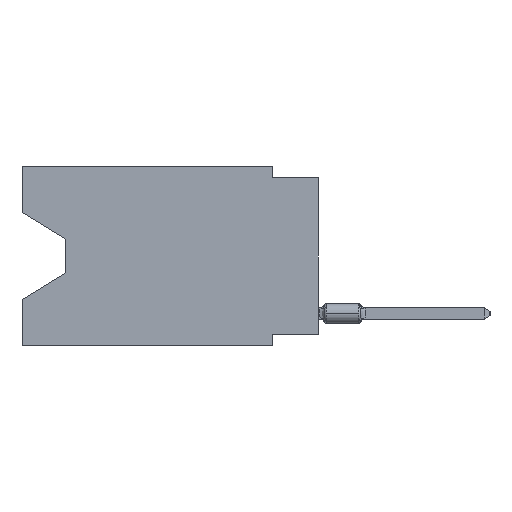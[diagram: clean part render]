
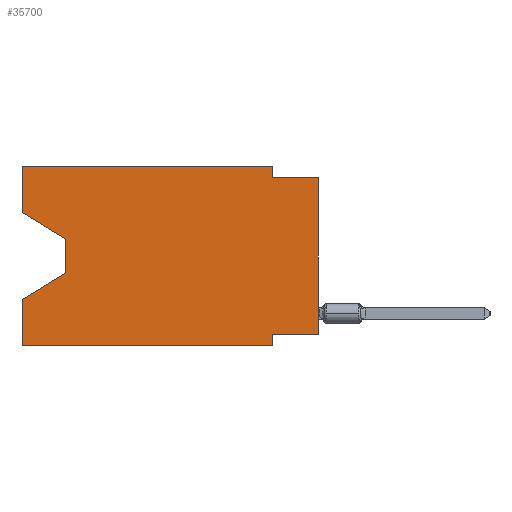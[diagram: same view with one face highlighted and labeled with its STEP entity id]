
A CAD part, left-side view. The second image highlights one B-rep face of the part: STEP entity #35700.
In plain terms, the highlighted planar face has unit normal (-1, 0, 0).
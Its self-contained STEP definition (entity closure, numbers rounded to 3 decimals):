
#218 = VERTEX_POINT ( 'NONE', #28616 ) ;
#376 = ORIENTED_EDGE ( 'NONE', *, *, #25564, .F. ) ;
#416 = CARTESIAN_POINT ( 'NONE',  ( 0., 2.54, -9.906 ) ) ;
#848 = LINE ( 'NONE', #58974, #63170 ) ;
#940 = DIRECTION ( 'NONE',  ( 0., -0.855, -0.519 ) ) ;
#2108 = VERTEX_POINT ( 'NONE', #58281 ) ;
#2671 = VERTEX_POINT ( 'NONE', #14211 ) ;
#4858 = CARTESIAN_POINT ( 'NONE',  ( 0., 13.97, -4.013 ) ) ;
#4919 = VECTOR ( 'NONE', #16366, 1000. ) ;
#5363 = DIRECTION ( 'NONE',  ( 0., 0., -1. ) ) ;
#5386 = LINE ( 'NONE', #6330, #28472 ) ;
#5789 = LINE ( 'NONE', #11554, #56213 ) ;
#6099 = CARTESIAN_POINT ( 'NONE',  ( 0., 0., 0. ) ) ;
#6330 = CARTESIAN_POINT ( 'NONE',  ( 0., 13.97, -5.893 ) ) ;
#7498 = VERTEX_POINT ( 'NONE', #21875 ) ;
#8392 = CARTESIAN_POINT ( 'NONE',  ( 0., 16.383, 0. ) ) ;
#8620 = ORIENTED_EDGE ( 'NONE', *, *, #43107, .F. ) ;
#8689 = ORIENTED_EDGE ( 'NONE', *, *, #15774, .T. ) ;
#9428 = CARTESIAN_POINT ( 'NONE',  ( 0., 2.54, 0. ) ) ;
#10363 = LINE ( 'NONE', #9428, #48111 ) ;
#10622 = CARTESIAN_POINT ( 'NONE',  ( 0., 16.383, 0. ) ) ;
#11326 = LINE ( 'NONE', #54697, #46266 ) ;
#11554 = CARTESIAN_POINT ( 'NONE',  ( 0., 0., -9.271 ) ) ;
#12272 = CARTESIAN_POINT ( 'NONE',  ( 0., 16.383, -9.906 ) ) ;
#13131 = CARTESIAN_POINT ( 'NONE',  ( 0., 16.383, -9.906 ) ) ;
#13269 = VERTEX_POINT ( 'NONE', #15925 ) ;
#13494 = CARTESIAN_POINT ( 'NONE',  ( 0., 0., -0.635 ) ) ;
#14211 = CARTESIAN_POINT ( 'NONE',  ( 0., 2.54, -0.635 ) ) ;
#14510 = LINE ( 'NONE', #4858, #38247 ) ;
#15774 = EDGE_CURVE ( 'NONE', #21392, #31409, #52078, .T. ) ;
#15925 = CARTESIAN_POINT ( 'NONE',  ( 0., 13.97, -4.013 ) ) ;
#16297 = VECTOR ( 'NONE', #37740, 1000. ) ;
#16366 = DIRECTION ( 'NONE',  ( 0., 0., 1. ) ) ;
#18761 = DIRECTION ( 'NONE',  ( 0., 0., -1. ) ) ;
#19205 = EDGE_CURVE ( 'NONE', #218, #7498, #5386, .T. ) ;
#20075 = ORIENTED_EDGE ( 'NONE', *, *, #20767, .F. ) ;
#20181 = EDGE_CURVE ( 'NONE', #2671, #57462, #52191, .T. ) ;
#20661 = PLANE ( 'NONE',  #23917 ) ;
#20767 = EDGE_CURVE ( 'NONE', #58159, #2671, #10363, .T. ) ;
#20881 = DIRECTION ( 'NONE',  ( 0., 1., 0. ) ) ;
#20971 = CARTESIAN_POINT ( 'NONE',  ( 0., 16.383, 0. ) ) ;
#21392 = VERTEX_POINT ( 'NONE', #13131 ) ;
#21606 = DIRECTION ( 'NONE',  ( 1., 0., 0. ) ) ;
#21875 = CARTESIAN_POINT ( 'NONE',  ( 0., 16.383, -7.36 ) ) ;
#23917 = AXIS2_PLACEMENT_3D ( 'NONE', #20971, #21606, #45676 ) ;
#24221 = ORIENTED_EDGE ( 'NONE', *, *, #39720, .F. ) ;
#25149 = EDGE_CURVE ( 'NONE', #21392, #7498, #11326, .T. ) ;
#25476 = DIRECTION ( 'NONE',  ( 0., 0., 1. ) ) ;
#25564 = EDGE_CURVE ( 'NONE', #48340, #2108, #49148, .T. ) ;
#27394 = ORIENTED_EDGE ( 'NONE', *, *, #43182, .T. ) ;
#28472 = VECTOR ( 'NONE', #54826, 1000. ) ;
#28616 = CARTESIAN_POINT ( 'NONE',  ( 0., 13.97, -5.893 ) ) ;
#29432 = ORIENTED_EDGE ( 'NONE', *, *, #40557, .T. ) ;
#29921 = VECTOR ( 'NONE', #53969, 1000. ) ;
#30432 = EDGE_CURVE ( 'NONE', #2108, #58159, #43688, .T. ) ;
#30510 = LINE ( 'NONE', #35319, #51999 ) ;
#31409 = VERTEX_POINT ( 'NONE', #416 ) ;
#31684 = EDGE_LOOP ( 'NONE', ( #29432, #59317, #34678, #61966, #8689, #24221, #8620, #27394, #58551, #20075, #40202, #376 ) ) ;
#34678 = ORIENTED_EDGE ( 'NONE', *, *, #19205, .T. ) ;
#34717 = CARTESIAN_POINT ( 'NONE',  ( 0., 0., -9.271 ) ) ;
#35319 = CARTESIAN_POINT ( 'NONE',  ( 0., 16.383, -2.546 ) ) ;
#35700 = ADVANCED_FACE ( 'NONE', ( #50807 ), #20661, .F. ) ;
#37158 = EDGE_CURVE ( 'NONE', #13269, #218, #14510, .T. ) ;
#37319 = DIRECTION ( 'NONE',  ( 0., -1., 0. ) ) ;
#37740 = DIRECTION ( 'NONE',  ( 0., -1., 0. ) ) ;
#38247 = VECTOR ( 'NONE', #43415, 1000. ) ;
#39720 = EDGE_CURVE ( 'NONE', #55018, #31409, #848, .T. ) ;
#40032 = CARTESIAN_POINT ( 'NONE',  ( 0., 2.54, 0. ) ) ;
#40202 = ORIENTED_EDGE ( 'NONE', *, *, #30432, .F. ) ;
#40557 = EDGE_CURVE ( 'NONE', #48340, #13269, #30510, .T. ) ;
#40761 = LINE ( 'NONE', #6099, #4919 ) ;
#42299 = CARTESIAN_POINT ( 'NONE',  ( 0., 2.54, -9.271 ) ) ;
#42604 = VECTOR ( 'NONE', #57843, 1000. ) ;
#43107 = EDGE_CURVE ( 'NONE', #61561, #55018, #5789, .T. ) ;
#43182 = EDGE_CURVE ( 'NONE', #61561, #57462, #40761, .T. ) ;
#43415 = DIRECTION ( 'NONE',  ( 0., 0., -1. ) ) ;
#43688 = LINE ( 'NONE', #8392, #42604 ) ;
#45676 = DIRECTION ( 'NONE',  ( 0., 0., -1. ) ) ;
#46266 = VECTOR ( 'NONE', #25476, 1000. ) ;
#48111 = VECTOR ( 'NONE', #18761, 1000. ) ;
#48340 = VERTEX_POINT ( 'NONE', #50586 ) ;
#49148 = LINE ( 'NONE', #10622, #29921 ) ;
#50586 = CARTESIAN_POINT ( 'NONE',  ( 0., 16.383, -2.546 ) ) ;
#50807 = FACE_OUTER_BOUND ( 'NONE', #31684, .T. ) ;
#51999 = VECTOR ( 'NONE', #940, 1000. ) ;
#52078 = LINE ( 'NONE', #12272, #53308 ) ;
#52191 = LINE ( 'NONE', #63076, #16297 ) ;
#53308 = VECTOR ( 'NONE', #37319, 1000. ) ;
#53969 = DIRECTION ( 'NONE',  ( 0., 0., 1. ) ) ;
#54697 = CARTESIAN_POINT ( 'NONE',  ( 0., 16.383, 0. ) ) ;
#54826 = DIRECTION ( 'NONE',  ( 0., 0.855, -0.519 ) ) ;
#55018 = VERTEX_POINT ( 'NONE', #42299 ) ;
#56213 = VECTOR ( 'NONE', #20881, 1000. ) ;
#57462 = VERTEX_POINT ( 'NONE', #13494 ) ;
#57843 = DIRECTION ( 'NONE',  ( 0., -1., 0. ) ) ;
#58159 = VERTEX_POINT ( 'NONE', #40032 ) ;
#58281 = CARTESIAN_POINT ( 'NONE',  ( 0., 16.383, 0. ) ) ;
#58551 = ORIENTED_EDGE ( 'NONE', *, *, #20181, .F. ) ;
#58974 = CARTESIAN_POINT ( 'NONE',  ( 0., 2.54, -9.906 ) ) ;
#59317 = ORIENTED_EDGE ( 'NONE', *, *, #37158, .T. ) ;
#61561 = VERTEX_POINT ( 'NONE', #34717 ) ;
#61966 = ORIENTED_EDGE ( 'NONE', *, *, #25149, .F. ) ;
#63076 = CARTESIAN_POINT ( 'NONE',  ( 0., 0., -0.635 ) ) ;
#63170 = VECTOR ( 'NONE', #5363, 1000. ) ;
